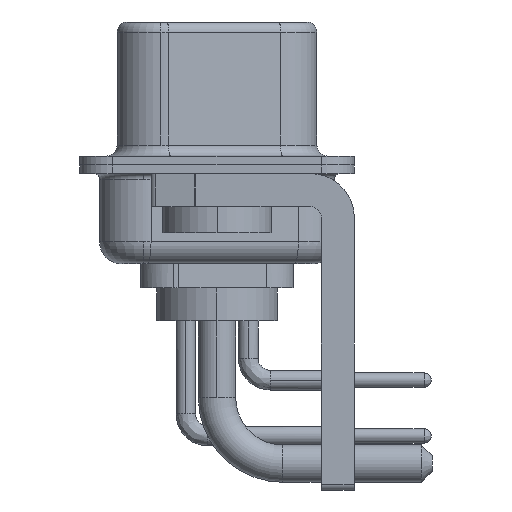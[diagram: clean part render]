
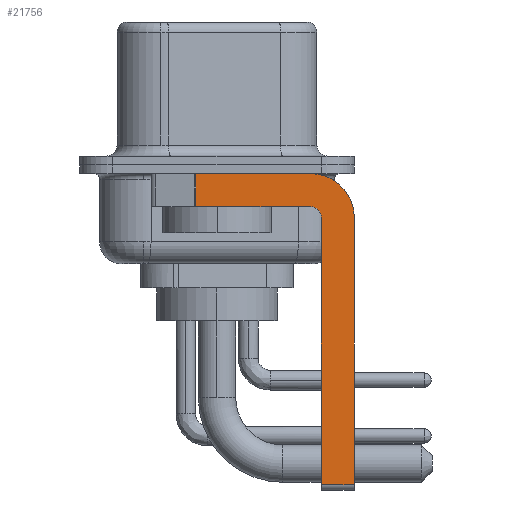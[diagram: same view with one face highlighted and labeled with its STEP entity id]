
A CAD part, left-side view. The second image highlights one B-rep face of the part: STEP entity #21756.
In plain terms, the highlighted planar face has unit normal (-1, 0, 0).
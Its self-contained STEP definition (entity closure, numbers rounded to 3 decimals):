
#397 = LINE ( 'NONE', #22849, #6566 ) ;
#464 = CARTESIAN_POINT ( 'NONE',  ( -2.9, 3., -0.4 ) ) ;
#602 = CARTESIAN_POINT ( 'NONE',  ( -2.9, -4.25, -2.4 ) ) ;
#1454 = DIRECTION ( 'NONE',  ( 0., 0., -1. ) ) ;
#2331 = ORIENTED_EDGE ( 'NONE', *, *, #4548, .F. ) ;
#2419 = LINE ( 'NONE', #16670, #21105 ) ;
#2751 = LINE ( 'NONE', #464, #22251 ) ;
#3155 = DIRECTION ( 'NONE',  ( 0., 0., 1. ) ) ;
#3913 = VERTEX_POINT ( 'NONE', #16887 ) ;
#4337 = DIRECTION ( 'NONE',  ( 0., 0., -1. ) ) ;
#4367 = EDGE_CURVE ( 'NONE', #18211, #23926, #2751, .T. ) ;
#4548 = EDGE_CURVE ( 'NONE', #5815, #5019, #21573, .T. ) ;
#5019 = VERTEX_POINT ( 'NONE', #7424 ) ;
#5294 = FACE_OUTER_BOUND ( 'NONE', #21079, .T. ) ;
#5303 = ORIENTED_EDGE ( 'NONE', *, *, #7267, .T. ) ;
#5716 = VERTEX_POINT ( 'NONE', #20639 ) ;
#5721 = VECTOR ( 'NONE', #1454, 1000. ) ;
#5815 = VERTEX_POINT ( 'NONE', #20774 ) ;
#6487 = CARTESIAN_POINT ( 'NONE',  ( -2.9, -4.25, -2.4 ) ) ;
#6566 = VECTOR ( 'NONE', #18539, 1000. ) ;
#7197 = CIRCLE ( 'NONE', #20938, 0.5 ) ;
#7267 = EDGE_CURVE ( 'NONE', #5815, #20778, #397, .T. ) ;
#7424 = CARTESIAN_POINT ( 'NONE',  ( -2.9, -4.75, -2.4 ) ) ;
#7549 = EDGE_CURVE ( 'NONE', #5716, #20778, #16444, .T. ) ;
#7561 = LINE ( 'NONE', #25983, #19026 ) ;
#8526 = ORIENTED_EDGE ( 'NONE', *, *, #25335, .T. ) ;
#8894 = ORIENTED_EDGE ( 'NONE', *, *, #7549, .F. ) ;
#9088 = AXIS2_PLACEMENT_3D ( 'NONE', #6487, #14421, #4337 ) ;
#9631 = ORIENTED_EDGE ( 'NONE', *, *, #4367, .F. ) ;
#10348 = DIRECTION ( 'NONE',  ( 0., 0., 1. ) ) ;
#10853 = CIRCLE ( 'NONE', #9088, 2. ) ;
#12514 = CARTESIAN_POINT ( 'NONE',  ( -2.9, 0.978, -0.4 ) ) ;
#12651 = ORIENTED_EDGE ( 'NONE', *, *, #18589, .F. ) ;
#13563 = CARTESIAN_POINT ( 'NONE',  ( -2.9, -4.25, -0.4 ) ) ;
#13838 = CARTESIAN_POINT ( 'NONE',  ( -2.9, -4.25, -2.4 ) ) ;
#14231 = DIRECTION ( 'NONE',  ( -1., 0., 0. ) ) ;
#14421 = DIRECTION ( 'NONE',  ( 1., 0., 0. ) ) ;
#14998 = DIRECTION ( 'NONE',  ( 0., -1., 0. ) ) ;
#15638 = CARTESIAN_POINT ( 'NONE',  ( -2.9, -4.25, -1.9 ) ) ;
#16179 = CARTESIAN_POINT ( 'NONE',  ( -2.9, -6.25, -2.4 ) ) ;
#16309 = ORIENTED_EDGE ( 'NONE', *, *, #23185, .F. ) ;
#16444 = LINE ( 'NONE', #16179, #5721 ) ;
#16670 = CARTESIAN_POINT ( 'NONE',  ( -2.9, -4.25, -1.9 ) ) ;
#16887 = CARTESIAN_POINT ( 'NONE',  ( -2.9, 0.978, -1.9 ) ) ;
#16994 = DIRECTION ( 'NONE',  ( 1., 0., 0. ) ) ;
#17528 = CARTESIAN_POINT ( 'NONE',  ( -2.9, -4.75, -14.8 ) ) ;
#17943 = VERTEX_POINT ( 'NONE', #15638 ) ;
#18211 = VERTEX_POINT ( 'NONE', #12514 ) ;
#18539 = DIRECTION ( 'NONE',  ( 0., -1., 0. ) ) ;
#18589 = EDGE_CURVE ( 'NONE', #5019, #17943, #7197, .T. ) ;
#19026 = VECTOR ( 'NONE', #24492, 1000. ) ;
#19027 = PLANE ( 'NONE',  #20249 ) ;
#19765 = CARTESIAN_POINT ( 'NONE',  ( -2.9, -6.25, -14.55 ) ) ;
#20249 = AXIS2_PLACEMENT_3D ( 'NONE', #602, #16994, #25225 ) ;
#20639 = CARTESIAN_POINT ( 'NONE',  ( -2.9, -6.25, -2.4 ) ) ;
#20774 = CARTESIAN_POINT ( 'NONE',  ( -2.9, -4.75, -14.55 ) ) ;
#20778 = VERTEX_POINT ( 'NONE', #19765 ) ;
#20938 = AXIS2_PLACEMENT_3D ( 'NONE', #13838, #14231, #10348 ) ;
#21079 = EDGE_LOOP ( 'NONE', ( #9631, #8526, #22567, #12651, #2331, #5303, #8894, #16309 ) ) ;
#21105 = VECTOR ( 'NONE', #24903, 1000. ) ;
#21573 = LINE ( 'NONE', #17528, #24495 ) ;
#21756 = ADVANCED_FACE ( 'NONE', ( #5294 ), #19027, .F. ) ;
#22251 = VECTOR ( 'NONE', #14998, 1000. ) ;
#22376 = EDGE_CURVE ( 'NONE', #17943, #3913, #2419, .T. ) ;
#22567 = ORIENTED_EDGE ( 'NONE', *, *, #22376, .F. ) ;
#22849 = CARTESIAN_POINT ( 'NONE',  ( -2.9, -4.25, -14.55 ) ) ;
#23185 = EDGE_CURVE ( 'NONE', #23926, #5716, #10853, .T. ) ;
#23926 = VERTEX_POINT ( 'NONE', #13563 ) ;
#24492 = DIRECTION ( 'NONE',  ( 0., 0., -1. ) ) ;
#24495 = VECTOR ( 'NONE', #3155, 1000. ) ;
#24903 = DIRECTION ( 'NONE',  ( 0., 1., 0. ) ) ;
#25225 = DIRECTION ( 'NONE',  ( 0., 0., -1. ) ) ;
#25335 = EDGE_CURVE ( 'NONE', #18211, #3913, #7561, .T. ) ;
#25983 = CARTESIAN_POINT ( 'NONE',  ( -2.9, 0.978, -1.9 ) ) ;
